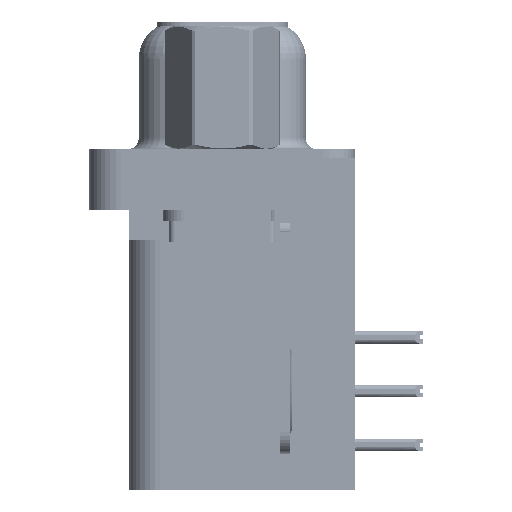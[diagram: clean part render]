
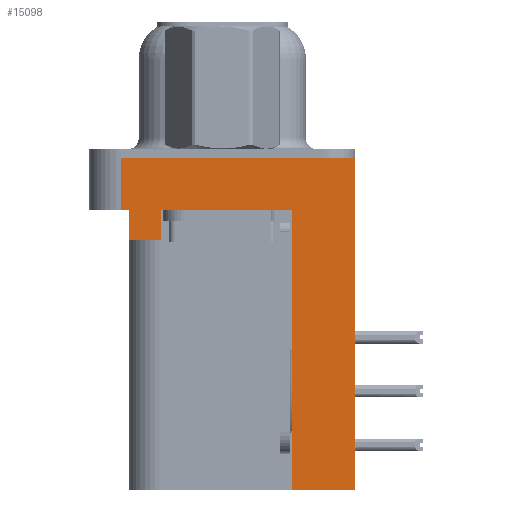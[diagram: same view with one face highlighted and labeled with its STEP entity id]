
A CAD part, left-side view. The second image highlights one B-rep face of the part: STEP entity #15098.
In plain terms, the highlighted planar face has unit normal (-1, 0, 0).
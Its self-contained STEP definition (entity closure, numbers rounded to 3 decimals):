
#80 = CARTESIAN_POINT ( 'NONE',  ( -3., -6.275, 0. ) ) ;
#276 = CARTESIAN_POINT ( 'NONE',  ( -3., -6.275, -2.5 ) ) ;
#375 = CARTESIAN_POINT ( 'NONE',  ( -3., 4.425, -3.9 ) ) ;
#498 = VERTEX_POINT ( 'NONE', #24803 ) ;
#1105 = DIRECTION ( 'NONE',  ( -1., 0., 0. ) ) ;
#1776 = EDGE_LOOP ( 'NONE', ( #32403, #34139, #6037, #47977, #21410, #23754, #4675, #29954, #22997, #37218 ) ) ;
#3469 = EDGE_CURVE ( 'NONE', #46893, #498, #36586, .T. ) ;
#3485 = VERTEX_POINT ( 'NONE', #80 ) ;
#3823 = EDGE_CURVE ( 'NONE', #22999, #3485, #25512, .T. ) ;
#4442 = CARTESIAN_POINT ( 'NONE',  ( -3., 4.775, -2.5 ) ) ;
#4675 = ORIENTED_EDGE ( 'NONE', *, *, #31763, .T. ) ;
#5762 = FACE_OUTER_BOUND ( 'NONE', #1776, .T. ) ;
#6037 = ORIENTED_EDGE ( 'NONE', *, *, #14974, .T. ) ;
#6998 = VECTOR ( 'NONE', #23935, 1000. ) ;
#7394 = LINE ( 'NONE', #36811, #7992 ) ;
#7763 = LINE ( 'NONE', #276, #6998 ) ;
#7887 = CARTESIAN_POINT ( 'NONE',  ( -3., -3.295, -15.7 ) ) ;
#7906 = DIRECTION ( 'NONE',  ( 0., 0., 1. ) ) ;
#7992 = VECTOR ( 'NONE', #16858, 1000. ) ;
#8588 = VERTEX_POINT ( 'NONE', #13634 ) ;
#9769 = VECTOR ( 'NONE', #26919, 1000. ) ;
#9901 = VECTOR ( 'NONE', #7906, 1000. ) ;
#9908 = LINE ( 'NONE', #47241, #9901 ) ;
#10024 = DIRECTION ( 'NONE',  ( 0., 0., 1. ) ) ;
#10293 = LINE ( 'NONE', #38750, #9769 ) ;
#11815 = DIRECTION ( 'NONE',  ( 0., 1., 0. ) ) ;
#13634 = CARTESIAN_POINT ( 'NONE',  ( -3., 2.895, -2.5 ) ) ;
#14974 = EDGE_CURVE ( 'NONE', #36965, #498, #7763, .T. ) ;
#15098 = ADVANCED_FACE ( 'NONE', ( #5762 ), #40682, .T. ) ;
#16858 = DIRECTION ( 'NONE',  ( 0., 0., 1. ) ) ;
#17632 = VERTEX_POINT ( 'NONE', #25220 ) ;
#18101 = DIRECTION ( 'NONE',  ( 0., -1., 0. ) ) ;
#19393 = CARTESIAN_POINT ( 'NONE',  ( -3., -6.275, 0. ) ) ;
#20954 = VECTOR ( 'NONE', #49612, 1000. ) ;
#21027 = CARTESIAN_POINT ( 'NONE',  ( -3., -6.275, -15.7 ) ) ;
#21410 = ORIENTED_EDGE ( 'NONE', *, *, #45922, .F. ) ;
#21483 = VERTEX_POINT ( 'NONE', #21027 ) ;
#22558 = LINE ( 'NONE', #45748, #20954 ) ;
#22997 = ORIENTED_EDGE ( 'NONE', *, *, #40775, .F. ) ;
#22999 = VERTEX_POINT ( 'NONE', #32544 ) ;
#23754 = ORIENTED_EDGE ( 'NONE', *, *, #38835, .T. ) ;
#23819 = VERTEX_POINT ( 'NONE', #45635 ) ;
#23935 = DIRECTION ( 'NONE',  ( 0., -1., 0. ) ) ;
#24439 = AXIS2_PLACEMENT_3D ( 'NONE', #44530, #1105, #28762 ) ;
#24543 = VERTEX_POINT ( 'NONE', #31034 ) ;
#24803 = CARTESIAN_POINT ( 'NONE',  ( -3., 4.425, -2.5 ) ) ;
#24907 = VECTOR ( 'NONE', #18101, 1000. ) ;
#25220 = CARTESIAN_POINT ( 'NONE',  ( -3., 2.895, -3.9 ) ) ;
#25512 = LINE ( 'NONE', #19393, #24907 ) ;
#26919 = DIRECTION ( 'NONE',  ( 0., -1., 0. ) ) ;
#28762 = DIRECTION ( 'NONE',  ( 0., 0., 1. ) ) ;
#29705 = CARTESIAN_POINT ( 'NONE',  ( -3., -6.275, -2.5 ) ) ;
#29954 = ORIENTED_EDGE ( 'NONE', *, *, #37926, .F. ) ;
#30760 = VECTOR ( 'NONE', #11815, 1000. ) ;
#31034 = CARTESIAN_POINT ( 'NONE',  ( -3., -3.295, -2.5 ) ) ;
#31053 = LINE ( 'NONE', #7887, #30760 ) ;
#31763 = EDGE_CURVE ( 'NONE', #8588, #24543, #10293, .T. ) ;
#32403 = ORIENTED_EDGE ( 'NONE', *, *, #3823, .F. ) ;
#32544 = CARTESIAN_POINT ( 'NONE',  ( -3., 4.775, 0. ) ) ;
#33137 = CARTESIAN_POINT ( 'NONE',  ( -3., 4.425, -3.9 ) ) ;
#34139 = ORIENTED_EDGE ( 'NONE', *, *, #38079, .F. ) ;
#36586 = LINE ( 'NONE', #33137, #36642 ) ;
#36642 = VECTOR ( 'NONE', #51007, 1000. ) ;
#36811 = CARTESIAN_POINT ( 'NONE',  ( -3., 4.775, -2.5 ) ) ;
#36965 = VERTEX_POINT ( 'NONE', #4442 ) ;
#37218 = ORIENTED_EDGE ( 'NONE', *, *, #38766, .T. ) ;
#37926 = EDGE_CURVE ( 'NONE', #23819, #24543, #9908, .T. ) ;
#38079 = EDGE_CURVE ( 'NONE', #36965, #22999, #7394, .T. ) ;
#38750 = CARTESIAN_POINT ( 'NONE',  ( -3., -6.275, -2.5 ) ) ;
#38766 = EDGE_CURVE ( 'NONE', #21483, #3485, #49313, .T. ) ;
#38835 = EDGE_CURVE ( 'NONE', #17632, #8588, #48868, .T. ) ;
#39470 = DIRECTION ( 'NONE',  ( 0., 0., 1. ) ) ;
#40682 = PLANE ( 'NONE',  #24439 ) ;
#40775 = EDGE_CURVE ( 'NONE', #21483, #23819, #31053, .T. ) ;
#42081 = CARTESIAN_POINT ( 'NONE',  ( -3., 2.895, -3.9 ) ) ;
#44530 = CARTESIAN_POINT ( 'NONE',  ( -3., -6.275, -2.5 ) ) ;
#45635 = CARTESIAN_POINT ( 'NONE',  ( -3., -3.295, -15.7 ) ) ;
#45748 = CARTESIAN_POINT ( 'NONE',  ( -3., 4.425, -3.9 ) ) ;
#45922 = EDGE_CURVE ( 'NONE', #17632, #46893, #22558, .T. ) ;
#46893 = VERTEX_POINT ( 'NONE', #375 ) ;
#47241 = CARTESIAN_POINT ( 'NONE',  ( -3., -3.295, -15.7 ) ) ;
#47977 = ORIENTED_EDGE ( 'NONE', *, *, #3469, .F. ) ;
#48868 = LINE ( 'NONE', #42081, #48882 ) ;
#48882 = VECTOR ( 'NONE', #39470, 1000. ) ;
#49267 = VECTOR ( 'NONE', #10024, 1000. ) ;
#49313 = LINE ( 'NONE', #29705, #49267 ) ;
#49612 = DIRECTION ( 'NONE',  ( 0., 1., 0. ) ) ;
#51007 = DIRECTION ( 'NONE',  ( 0., 0., 1. ) ) ;
